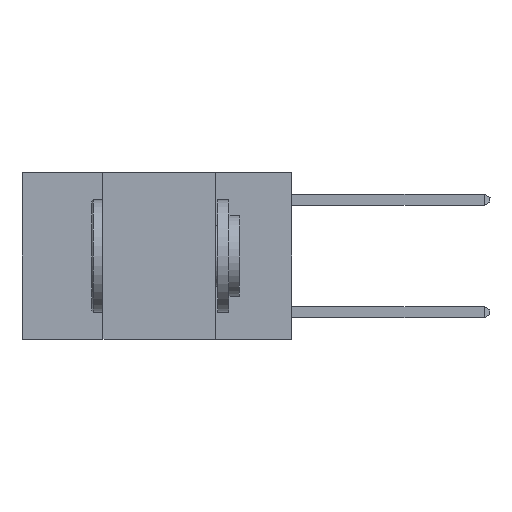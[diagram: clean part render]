
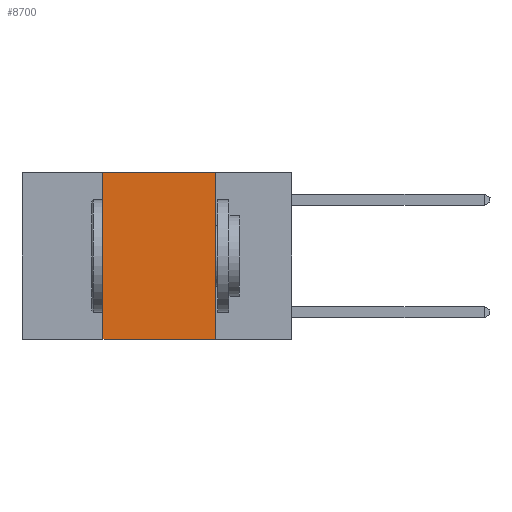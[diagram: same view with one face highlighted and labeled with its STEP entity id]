
A CAD part, left-side view. The second image highlights one B-rep face of the part: STEP entity #8700.
In plain terms, the highlighted planar face has unit normal (-1, 0, 0).
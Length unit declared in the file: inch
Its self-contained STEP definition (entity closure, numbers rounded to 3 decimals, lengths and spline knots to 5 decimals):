
#237 = CARTESIAN_POINT ( 'NONE',  ( 0., 0.42, -0.37 ) ) ;
#520 = DIRECTION ( 'NONE',  ( 0., 0., -1. ) ) ;
#836 = CARTESIAN_POINT ( 'NONE',  ( 0., 0.6, 0. ) ) ;
#1250 = LINE ( 'NONE', #10738, #10990 ) ;
#1802 = CARTESIAN_POINT ( 'NONE',  ( 0., 0.42, 0. ) ) ;
#1916 = EDGE_CURVE ( 'NONE', #7390, #2990, #8971, .T. ) ;
#2543 = EDGE_CURVE ( 'NONE', #7390, #6445, #7875, .T. ) ;
#2990 = VERTEX_POINT ( 'NONE', #4164 ) ;
#3134 = ORIENTED_EDGE ( 'NONE', *, *, #1916, .T. ) ;
#4123 = CARTESIAN_POINT ( 'NONE',  ( 0., 0.17, 0. ) ) ;
#4164 = CARTESIAN_POINT ( 'NONE',  ( 0., 0.17, -0.37 ) ) ;
#4203 = EDGE_CURVE ( 'NONE', #6445, #10613, #8273, .T. ) ;
#4376 = DIRECTION ( 'NONE',  ( 1., 0., 0. ) ) ;
#4711 = CARTESIAN_POINT ( 'NONE',  ( 0., 0.6, -0.37 ) ) ;
#5049 = ORIENTED_EDGE ( 'NONE', *, *, #2543, .F. ) ;
#5231 = VECTOR ( 'NONE', #9868, 39.37008 ) ;
#5740 = ORIENTED_EDGE ( 'NONE', *, *, #8813, .F. ) ;
#6099 = ORIENTED_EDGE ( 'NONE', *, *, #4203, .F. ) ;
#6445 = VERTEX_POINT ( 'NONE', #10159 ) ;
#6667 = VECTOR ( 'NONE', #7817, 39.37008 ) ;
#6852 = VECTOR ( 'NONE', #7634, 39.37008 ) ;
#7192 = EDGE_LOOP ( 'NONE', ( #5740, #6099, #5049, #3134 ) ) ;
#7216 = AXIS2_PLACEMENT_3D ( 'NONE', #9706, #4376, #8748 ) ;
#7390 = VERTEX_POINT ( 'NONE', #237 ) ;
#7634 = DIRECTION ( 'NONE',  ( 0., -1., 0. ) ) ;
#7817 = DIRECTION ( 'NONE',  ( 0., 0., 1. ) ) ;
#7875 = LINE ( 'NONE', #1802, #6667 ) ;
#8273 = LINE ( 'NONE', #836, #6852 ) ;
#8700 = ADVANCED_FACE ( 'NONE', ( #8862 ), #9601, .F. ) ;
#8748 = DIRECTION ( 'NONE',  ( 0., 0., -1. ) ) ;
#8813 = EDGE_CURVE ( 'NONE', #10613, #2990, #1250, .T. ) ;
#8862 = FACE_OUTER_BOUND ( 'NONE', #7192, .T. ) ;
#8971 = LINE ( 'NONE', #4711, #5231 ) ;
#9601 = PLANE ( 'NONE',  #7216 ) ;
#9706 = CARTESIAN_POINT ( 'NONE',  ( 0., 0.6, 0. ) ) ;
#9868 = DIRECTION ( 'NONE',  ( 0., -1., 0. ) ) ;
#10159 = CARTESIAN_POINT ( 'NONE',  ( 0., 0.42, 0. ) ) ;
#10613 = VERTEX_POINT ( 'NONE', #4123 ) ;
#10738 = CARTESIAN_POINT ( 'NONE',  ( 0., 0.17, 0. ) ) ;
#10990 = VECTOR ( 'NONE', #520, 39.37008 ) ;
